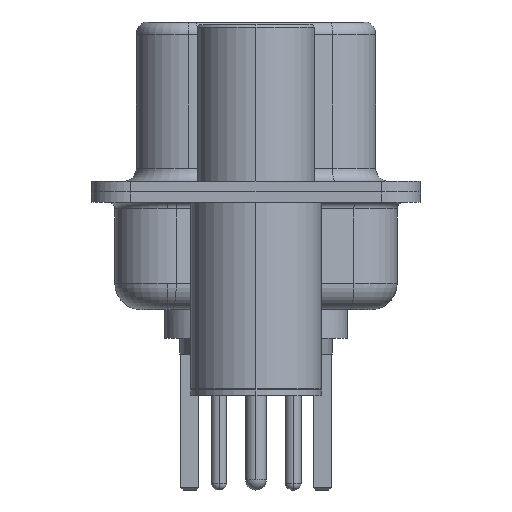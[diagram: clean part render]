
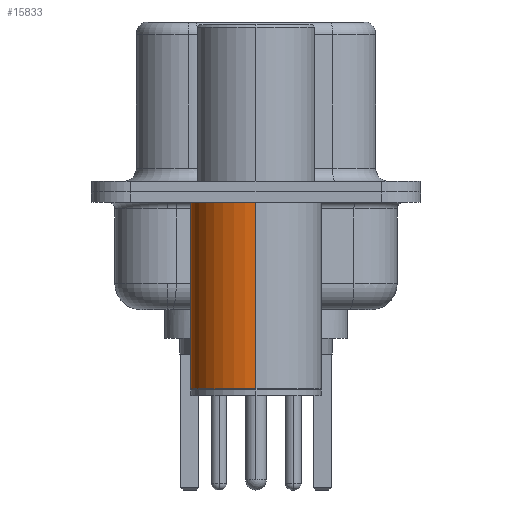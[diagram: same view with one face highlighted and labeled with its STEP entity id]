
A CAD part, left-side view. The second image highlights one B-rep face of the part: STEP entity #15833.
In plain terms, the highlighted cylindrical face has radius 2.5 mm (diameter 5 mm), a partial arc.
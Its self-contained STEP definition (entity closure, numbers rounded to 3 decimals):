
#423 = DIRECTION ( 'NONE',  ( 0., 0., 1. ) ) ;
#426 = ORIENTED_EDGE ( 'NONE', *, *, #11368, .T. ) ;
#430 = VERTEX_POINT ( 'NONE', #9813 ) ;
#2276 = VERTEX_POINT ( 'NONE', #10114 ) ;
#2672 = EDGE_CURVE ( 'NONE', #20919, #430, #3903, .T. ) ;
#3165 = CARTESIAN_POINT ( 'NONE',  ( 0., 0., 0.581 ) ) ;
#3380 = VECTOR ( 'NONE', #7532, 1000. ) ;
#3903 = LINE ( 'NONE', #21324, #3380 ) ;
#3963 = CIRCLE ( 'NONE', #12573, 2.5 ) ;
#4360 = EDGE_LOOP ( 'NONE', ( #7128, #426, #9787, #9019 ) ) ;
#4784 = LINE ( 'NONE', #12232, #13149 ) ;
#4836 = VERTEX_POINT ( 'NONE', #5583 ) ;
#5499 = CYLINDRICAL_SURFACE ( 'NONE', #5827, 2.5 ) ;
#5530 = DIRECTION ( 'NONE',  ( 0., 0., 1. ) ) ;
#5583 = CARTESIAN_POINT ( 'NONE',  ( -2.5, 0., -0.4 ) ) ;
#5827 = AXIS2_PLACEMENT_3D ( 'NONE', #3165, #6495, #11500 ) ;
#6495 = DIRECTION ( 'NONE',  ( 0., 0., 1. ) ) ;
#7128 = ORIENTED_EDGE ( 'NONE', *, *, #9941, .T. ) ;
#7532 = DIRECTION ( 'NONE',  ( 0., 0., 1. ) ) ;
#8860 = DIRECTION ( 'NONE',  ( 0., 0., 1. ) ) ;
#9019 = ORIENTED_EDGE ( 'NONE', *, *, #2672, .F. ) ;
#9787 = ORIENTED_EDGE ( 'NONE', *, *, #16034, .F. ) ;
#9813 = CARTESIAN_POINT ( 'NONE',  ( 2.5, 0., -0.4 ) ) ;
#9941 = EDGE_CURVE ( 'NONE', #20919, #2276, #10858, .T. ) ;
#10114 = CARTESIAN_POINT ( 'NONE',  ( -2.5, 0., -7.525 ) ) ;
#10385 = CARTESIAN_POINT ( 'NONE',  ( 0., 0., -7.525 ) ) ;
#10858 = CIRCLE ( 'NONE', #19248, 2.5 ) ;
#11368 = EDGE_CURVE ( 'NONE', #2276, #4836, #4784, .T. ) ;
#11500 = DIRECTION ( 'NONE',  ( 1., 0., 0. ) ) ;
#12058 = DIRECTION ( 'NONE',  ( 1., 0., 0. ) ) ;
#12232 = CARTESIAN_POINT ( 'NONE',  ( -2.5, 0., 0.581 ) ) ;
#12573 = AXIS2_PLACEMENT_3D ( 'NONE', #15515, #5530, #17195 ) ;
#13149 = VECTOR ( 'NONE', #8860, 1000. ) ;
#14871 = FACE_OUTER_BOUND ( 'NONE', #4360, .T. ) ;
#15515 = CARTESIAN_POINT ( 'NONE',  ( 0., 0., -0.4 ) ) ;
#15833 = ADVANCED_FACE ( 'NONE', ( #14871 ), #5499, .T. ) ;
#16034 = EDGE_CURVE ( 'NONE', #430, #4836, #3963, .T. ) ;
#17195 = DIRECTION ( 'NONE',  ( 1., 0., 0. ) ) ;
#18403 = CARTESIAN_POINT ( 'NONE',  ( 2.5, 0., -7.525 ) ) ;
#19248 = AXIS2_PLACEMENT_3D ( 'NONE', #10385, #423, #12058 ) ;
#20919 = VERTEX_POINT ( 'NONE', #18403 ) ;
#21324 = CARTESIAN_POINT ( 'NONE',  ( 2.5, 0., 0.581 ) ) ;
